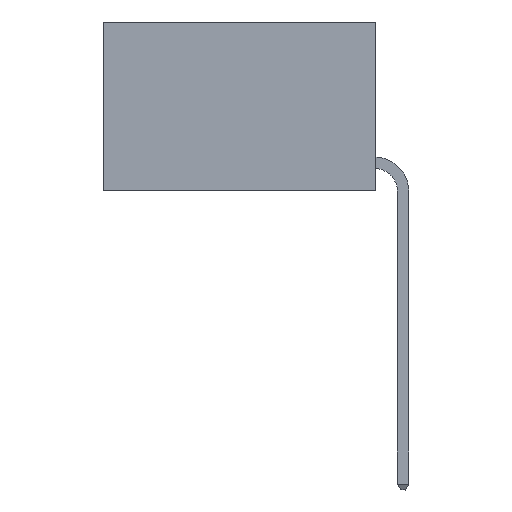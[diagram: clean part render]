
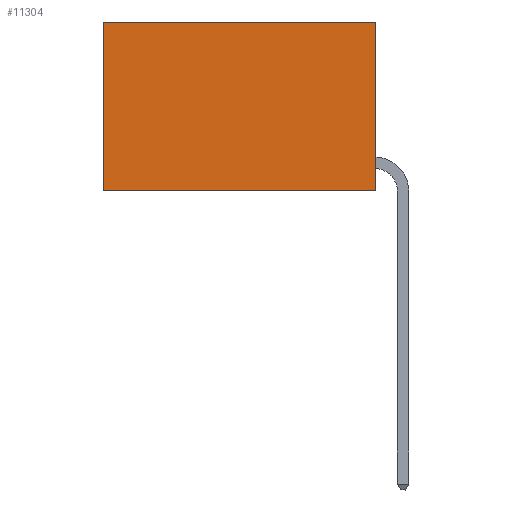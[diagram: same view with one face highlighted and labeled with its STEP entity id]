
A CAD part, left-side view. The second image highlights one B-rep face of the part: STEP entity #11304.
In plain terms, the highlighted planar face has unit normal (-1, 0, 0).
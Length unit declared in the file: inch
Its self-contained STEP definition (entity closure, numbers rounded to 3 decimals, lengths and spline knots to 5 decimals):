
#124 = CARTESIAN_POINT ( 'NONE',  ( 0.2625, 0.6, 0. ) ) ;
#216 = EDGE_CURVE ( 'NONE', #425, #15110, #19619, .T. ) ;
#425 = VERTEX_POINT ( 'NONE', #12412 ) ;
#628 = EDGE_CURVE ( 'NONE', #18965, #425, #18507, .T. ) ;
#1132 = CARTESIAN_POINT ( 'NONE',  ( 0.2625, 0.6, 0. ) ) ;
#1532 = DIRECTION ( 'NONE',  ( 1., 0., 0. ) ) ;
#2683 = EDGE_LOOP ( 'NONE', ( #19917, #8818, #16731, #7479 ) ) ;
#2843 = VECTOR ( 'NONE', #10771, 39.37008 ) ;
#4570 = CARTESIAN_POINT ( 'NONE',  ( 0.2625, 0., 0. ) ) ;
#4669 = AXIS2_PLACEMENT_3D ( 'NONE', #4570, #1532, #10753 ) ;
#4853 = DIRECTION ( 'NONE',  ( 0., 0., -1. ) ) ;
#7479 = ORIENTED_EDGE ( 'NONE', *, *, #14647, .T. ) ;
#7586 = FACE_OUTER_BOUND ( 'NONE', #2683, .T. ) ;
#7781 = EDGE_CURVE ( 'NONE', #13987, #15110, #12461, .T. ) ;
#7975 = VECTOR ( 'NONE', #4853, 39.37008 ) ;
#8753 = DIRECTION ( 'NONE',  ( 0., 1., 0. ) ) ;
#8818 = ORIENTED_EDGE ( 'NONE', *, *, #216, .F. ) ;
#9355 = CARTESIAN_POINT ( 'NONE',  ( 0.2625, 0., 0. ) ) ;
#9387 = CARTESIAN_POINT ( 'NONE',  ( 0.2625, 0., 0. ) ) ;
#9469 = VECTOR ( 'NONE', #12418, 39.37008 ) ;
#10753 = DIRECTION ( 'NONE',  ( 0., 0., -1. ) ) ;
#10771 = DIRECTION ( 'NONE',  ( 0., 1., 0. ) ) ;
#11304 = ADVANCED_FACE ( 'NONE', ( #7586 ), #18479, .F. ) ;
#12304 = LINE ( 'NONE', #18496, #2843 ) ;
#12412 = CARTESIAN_POINT ( 'NONE',  ( 0.2625, 0., -0.37 ) ) ;
#12418 = DIRECTION ( 'NONE',  ( 0., 0., -1. ) ) ;
#12461 = LINE ( 'NONE', #124, #7975 ) ;
#13987 = VERTEX_POINT ( 'NONE', #1132 ) ;
#14647 = EDGE_CURVE ( 'NONE', #18965, #13987, #12304, .T. ) ;
#15110 = VERTEX_POINT ( 'NONE', #19915 ) ;
#15958 = VECTOR ( 'NONE', #8753, 39.37008 ) ;
#16731 = ORIENTED_EDGE ( 'NONE', *, *, #628, .F. ) ;
#18086 = CARTESIAN_POINT ( 'NONE',  ( 0.2625, 0., -0.37 ) ) ;
#18479 = PLANE ( 'NONE',  #4669 ) ;
#18496 = CARTESIAN_POINT ( 'NONE',  ( 0.2625, 0., 0. ) ) ;
#18507 = LINE ( 'NONE', #9355, #9469 ) ;
#18965 = VERTEX_POINT ( 'NONE', #9387 ) ;
#19619 = LINE ( 'NONE', #18086, #15958 ) ;
#19915 = CARTESIAN_POINT ( 'NONE',  ( 0.2625, 0.6, -0.37 ) ) ;
#19917 = ORIENTED_EDGE ( 'NONE', *, *, #7781, .T. ) ;
